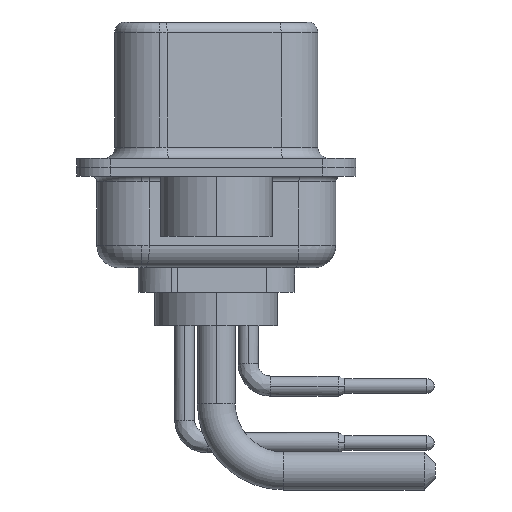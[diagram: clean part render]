
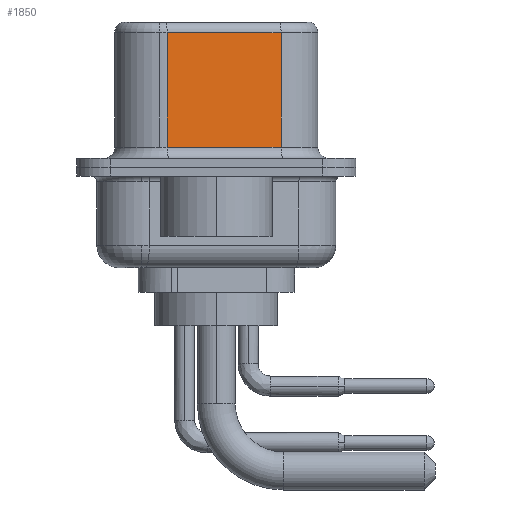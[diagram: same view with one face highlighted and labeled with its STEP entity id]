
A CAD part, left-side view. The second image highlights one B-rep face of the part: STEP entity #1850.
In plain terms, the highlighted planar face has unit normal (-0.985, -0.174, 0).
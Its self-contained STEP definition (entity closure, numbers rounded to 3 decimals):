
#802 = EDGE_CURVE ( 'NONE', #16344, #3694, #2740, .T. ) ;
#1850 = ADVANCED_FACE ( 'NONE', ( #19223 ), #11046, .F. ) ;
#2740 = LINE ( 'NONE', #7825, #11995 ) ;
#2878 = CARTESIAN_POINT ( 'NONE',  ( 4.555, -2.897, 6.52 ) ) ;
#3694 = VERTEX_POINT ( 'NONE', #8735 ) ;
#4363 = LINE ( 'NONE', #2878, #16289 ) ;
#4375 = ORIENTED_EDGE ( 'NONE', *, *, #11777, .T. ) ;
#5105 = ORIENTED_EDGE ( 'NONE', *, *, #6868, .F. ) ;
#5270 = EDGE_LOOP ( 'NONE', ( #5105, #4375, #15816, #8106 ) ) ;
#5564 = VERTEX_POINT ( 'NONE', #5951 ) ;
#5951 = CARTESIAN_POINT ( 'NONE',  ( 3.655, 2.203, 6.02 ) ) ;
#6160 = AXIS2_PLACEMENT_3D ( 'NONE', #17429, #15842, #20699 ) ;
#6237 = DIRECTION ( 'NONE',  ( 0.174, -0.985, 0. ) ) ;
#6534 = CARTESIAN_POINT ( 'NONE',  ( 3.655, 2.203, 0.9 ) ) ;
#6868 = EDGE_CURVE ( 'NONE', #7852, #3694, #4363, .T. ) ;
#7796 = LINE ( 'NONE', #19471, #10276 ) ;
#7825 = CARTESIAN_POINT ( 'NONE',  ( 4.555, -2.897, 0.9 ) ) ;
#7852 = VERTEX_POINT ( 'NONE', #16360 ) ;
#8106 = ORIENTED_EDGE ( 'NONE', *, *, #802, .T. ) ;
#8735 = CARTESIAN_POINT ( 'NONE',  ( 4.555, -2.897, 0.9 ) ) ;
#9809 = DIRECTION ( 'NONE',  ( -0.174, 0.985, 0. ) ) ;
#10276 = VECTOR ( 'NONE', #9809, 1000. ) ;
#11046 = PLANE ( 'NONE',  #6160 ) ;
#11049 = DIRECTION ( 'NONE',  ( 0., 0., -1. ) ) ;
#11424 = VECTOR ( 'NONE', #13788, 1000. ) ;
#11777 = EDGE_CURVE ( 'NONE', #7852, #5564, #7796, .T. ) ;
#11901 = CARTESIAN_POINT ( 'NONE',  ( 3.655, 2.203, 6.52 ) ) ;
#11995 = VECTOR ( 'NONE', #6237, 1000. ) ;
#13788 = DIRECTION ( 'NONE',  ( 0., 0., -1. ) ) ;
#15550 = EDGE_CURVE ( 'NONE', #5564, #16344, #20259, .T. ) ;
#15816 = ORIENTED_EDGE ( 'NONE', *, *, #15550, .T. ) ;
#15842 = DIRECTION ( 'NONE',  ( 0.985, 0.174, 0. ) ) ;
#16289 = VECTOR ( 'NONE', #11049, 1000. ) ;
#16344 = VERTEX_POINT ( 'NONE', #6534 ) ;
#16360 = CARTESIAN_POINT ( 'NONE',  ( 4.555, -2.897, 6.02 ) ) ;
#17429 = CARTESIAN_POINT ( 'NONE',  ( 4.555, -2.897, 6.52 ) ) ;
#19223 = FACE_OUTER_BOUND ( 'NONE', #5270, .T. ) ;
#19471 = CARTESIAN_POINT ( 'NONE',  ( 4.555, -2.897, 6.02 ) ) ;
#20259 = LINE ( 'NONE', #11901, #11424 ) ;
#20699 = DIRECTION ( 'NONE',  ( -0.174, 0.985, 0. ) ) ;
